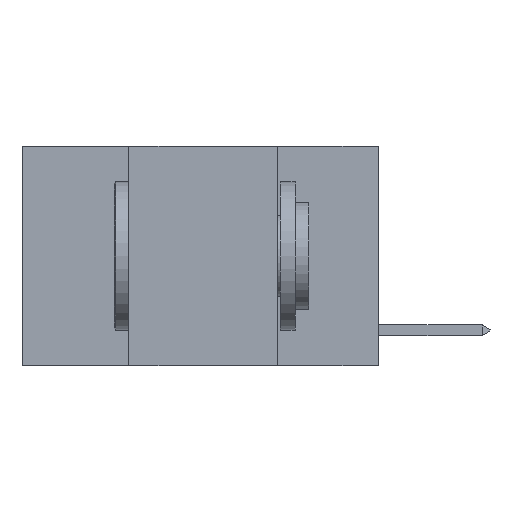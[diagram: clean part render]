
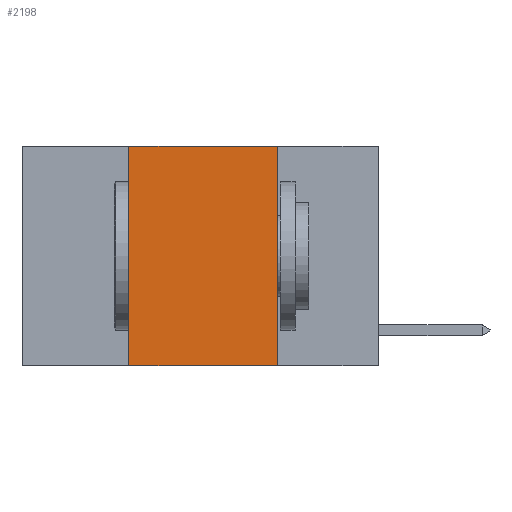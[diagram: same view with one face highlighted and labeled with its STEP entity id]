
A CAD part, left-side view. The second image highlights one B-rep face of the part: STEP entity #2198.
In plain terms, the highlighted planar face has unit normal (-1, 0, 0).
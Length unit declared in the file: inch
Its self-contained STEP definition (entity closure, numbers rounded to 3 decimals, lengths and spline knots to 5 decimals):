
#94 = CARTESIAN_POINT ( 'NONE',  ( 0., 0.42, 0. ) ) ;
#817 = CARTESIAN_POINT ( 'NONE',  ( 0., 0.17, -0.37 ) ) ;
#826 = VERTEX_POINT ( 'NONE', #94 ) ;
#1018 = EDGE_CURVE ( 'NONE', #2937, #826, #2456, .T. ) ;
#1451 = FACE_OUTER_BOUND ( 'NONE', #9733, .T. ) ;
#1809 = ORIENTED_EDGE ( 'NONE', *, *, #4030, .F. ) ;
#2198 = ADVANCED_FACE ( 'NONE', ( #1451 ), #3021, .F. ) ;
#2236 = DIRECTION ( 'NONE',  ( 1., 0., 0. ) ) ;
#2456 = LINE ( 'NONE', #6522, #4434 ) ;
#2937 = VERTEX_POINT ( 'NONE', #7966 ) ;
#3021 = PLANE ( 'NONE',  #5252 ) ;
#4030 = EDGE_CURVE ( 'NONE', #826, #7990, #5196, .T. ) ;
#4434 = VECTOR ( 'NONE', #8014, 39.37008 ) ;
#4451 = CARTESIAN_POINT ( 'NONE',  ( 0., 0.6, 0. ) ) ;
#4722 = DIRECTION ( 'NONE',  ( 0., 0., -1. ) ) ;
#4999 = CARTESIAN_POINT ( 'NONE',  ( 0., 0.17, 0. ) ) ;
#5196 = LINE ( 'NONE', #4451, #8225 ) ;
#5252 = AXIS2_PLACEMENT_3D ( 'NONE', #7997, #2236, #8694 ) ;
#5289 = ORIENTED_EDGE ( 'NONE', *, *, #1018, .F. ) ;
#5342 = VERTEX_POINT ( 'NONE', #817 ) ;
#6522 = CARTESIAN_POINT ( 'NONE',  ( 0., 0.42, 0. ) ) ;
#6556 = ORIENTED_EDGE ( 'NONE', *, *, #6870, .F. ) ;
#6829 = CARTESIAN_POINT ( 'NONE',  ( 0., 0.6, -0.37 ) ) ;
#6870 = EDGE_CURVE ( 'NONE', #7990, #5342, #10367, .T. ) ;
#6998 = CARTESIAN_POINT ( 'NONE',  ( 0., 0.17, 0. ) ) ;
#7053 = EDGE_CURVE ( 'NONE', #2937, #5342, #9204, .T. ) ;
#7181 = ORIENTED_EDGE ( 'NONE', *, *, #7053, .T. ) ;
#7208 = VECTOR ( 'NONE', #4722, 39.37008 ) ;
#7966 = CARTESIAN_POINT ( 'NONE',  ( 0., 0.42, -0.37 ) ) ;
#7990 = VERTEX_POINT ( 'NONE', #4999 ) ;
#7997 = CARTESIAN_POINT ( 'NONE',  ( 0., 0.6, 0. ) ) ;
#8014 = DIRECTION ( 'NONE',  ( 0., 0., 1. ) ) ;
#8225 = VECTOR ( 'NONE', #8662, 39.37008 ) ;
#8424 = DIRECTION ( 'NONE',  ( 0., -1., 0. ) ) ;
#8662 = DIRECTION ( 'NONE',  ( 0., -1., 0. ) ) ;
#8694 = DIRECTION ( 'NONE',  ( 0., 0., -1. ) ) ;
#9204 = LINE ( 'NONE', #6829, #9855 ) ;
#9733 = EDGE_LOOP ( 'NONE', ( #6556, #1809, #5289, #7181 ) ) ;
#9855 = VECTOR ( 'NONE', #8424, 39.37008 ) ;
#10367 = LINE ( 'NONE', #6998, #7208 ) ;
